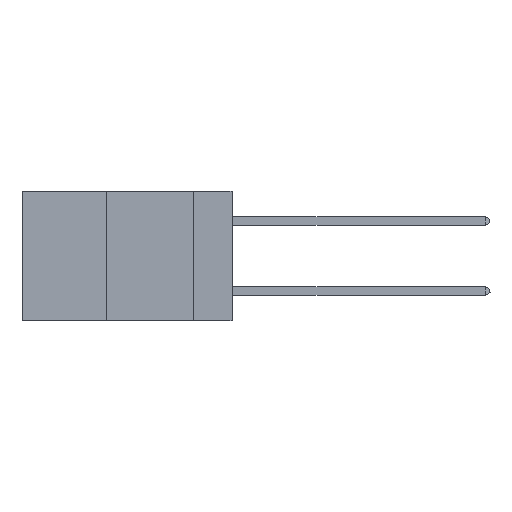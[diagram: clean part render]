
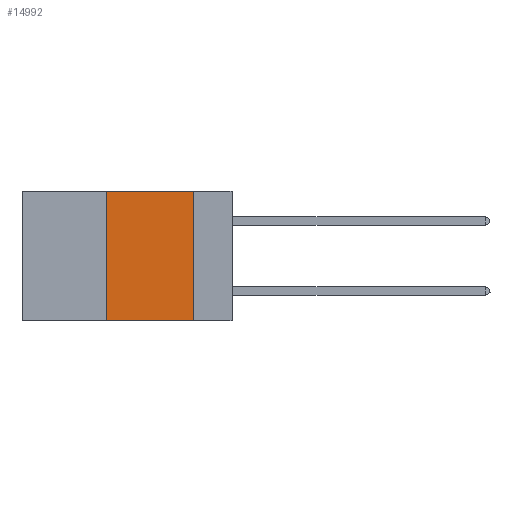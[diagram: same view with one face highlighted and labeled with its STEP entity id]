
A CAD part, left-side view. The second image highlights one B-rep face of the part: STEP entity #14992.
In plain terms, the highlighted planar face has unit normal (-1, 0, 0).
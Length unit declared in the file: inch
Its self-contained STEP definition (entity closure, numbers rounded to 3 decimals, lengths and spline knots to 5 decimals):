
#247 = CARTESIAN_POINT ( 'NONE',  ( 0., 0.36, 0. ) ) ;
#268 = VERTEX_POINT ( 'NONE', #3114 ) ;
#1125 = CARTESIAN_POINT ( 'NONE',  ( 0., 0.6, 0. ) ) ;
#1745 = CARTESIAN_POINT ( 'NONE',  ( 0., 0.6, 0. ) ) ;
#1853 = EDGE_CURVE ( 'NONE', #15260, #13054, #5127, .T. ) ;
#1948 = VECTOR ( 'NONE', #3313, 39.37008 ) ;
#2396 = DIRECTION ( 'NONE',  ( 0., 0., -1. ) ) ;
#2958 = DIRECTION ( 'NONE',  ( 0., -1., 0. ) ) ;
#3114 = CARTESIAN_POINT ( 'NONE',  ( 0., 0.11, -0.37 ) ) ;
#3313 = DIRECTION ( 'NONE',  ( 0., 0., -1. ) ) ;
#4321 = EDGE_CURVE ( 'NONE', #15260, #268, #6483, .T. ) ;
#4824 = LINE ( 'NONE', #11681, #1948 ) ;
#5121 = ORIENTED_EDGE ( 'NONE', *, *, #13324, .F. ) ;
#5127 = LINE ( 'NONE', #7294, #11051 ) ;
#5480 = ORIENTED_EDGE ( 'NONE', *, *, #4321, .T. ) ;
#6483 = LINE ( 'NONE', #10108, #15393 ) ;
#7226 = PLANE ( 'NONE',  #13170 ) ;
#7294 = CARTESIAN_POINT ( 'NONE',  ( 0., 0.36, 0. ) ) ;
#7540 = VECTOR ( 'NONE', #7826, 39.37008 ) ;
#7826 = DIRECTION ( 'NONE',  ( 0., -1., 0. ) ) ;
#8271 = ORIENTED_EDGE ( 'NONE', *, *, #10905, .F. ) ;
#8718 = EDGE_LOOP ( 'NONE', ( #5121, #8271, #11404, #5480 ) ) ;
#8805 = CARTESIAN_POINT ( 'NONE',  ( 0., 0.36, -0.37 ) ) ;
#9597 = DIRECTION ( 'NONE',  ( 1., 0., 0. ) ) ;
#10108 = CARTESIAN_POINT ( 'NONE',  ( 0., 0.6, -0.37 ) ) ;
#10279 = VERTEX_POINT ( 'NONE', #11444 ) ;
#10642 = LINE ( 'NONE', #1745, #7540 ) ;
#10905 = EDGE_CURVE ( 'NONE', #13054, #10279, #10642, .T. ) ;
#11051 = VECTOR ( 'NONE', #12508, 39.37008 ) ;
#11404 = ORIENTED_EDGE ( 'NONE', *, *, #1853, .F. ) ;
#11444 = CARTESIAN_POINT ( 'NONE',  ( 0., 0.11, 0. ) ) ;
#11681 = CARTESIAN_POINT ( 'NONE',  ( 0., 0.11, 0. ) ) ;
#12508 = DIRECTION ( 'NONE',  ( 0., 0., 1. ) ) ;
#13054 = VERTEX_POINT ( 'NONE', #247 ) ;
#13170 = AXIS2_PLACEMENT_3D ( 'NONE', #1125, #9597, #2396 ) ;
#13324 = EDGE_CURVE ( 'NONE', #10279, #268, #4824, .T. ) ;
#14602 = FACE_OUTER_BOUND ( 'NONE', #8718, .T. ) ;
#14992 = ADVANCED_FACE ( 'NONE', ( #14602 ), #7226, .F. ) ;
#15260 = VERTEX_POINT ( 'NONE', #8805 ) ;
#15393 = VECTOR ( 'NONE', #2958, 39.37008 ) ;
